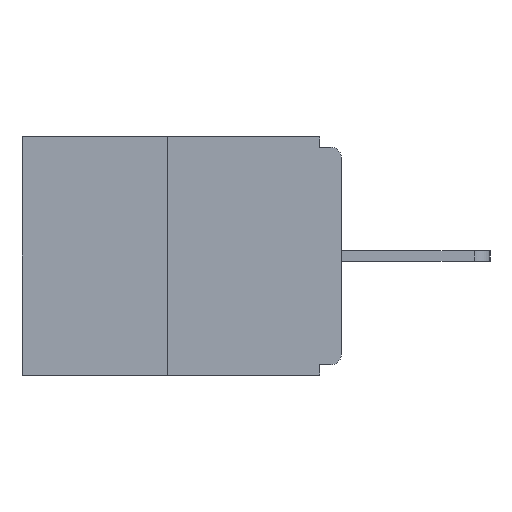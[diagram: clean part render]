
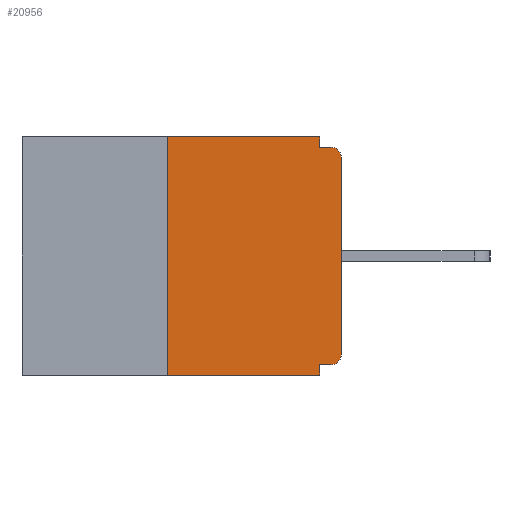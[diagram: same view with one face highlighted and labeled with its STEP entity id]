
A CAD part, left-side view. The second image highlights one B-rep face of the part: STEP entity #20956.
In plain terms, the highlighted planar face has unit normal (-1, 0, 0).
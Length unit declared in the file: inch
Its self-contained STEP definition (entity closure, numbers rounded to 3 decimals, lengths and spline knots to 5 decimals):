
#208 = PLANE ( 'NONE',  #18270 ) ;
#261 = ORIENTED_EDGE ( 'NONE', *, *, #8516, .T. ) ;
#302 = DIRECTION ( 'NONE',  ( 0., 0., -1. ) ) ;
#367 = VERTEX_POINT ( 'NONE', #8144 ) ;
#440 = DIRECTION ( 'NONE',  ( -1., 0., 0. ) ) ;
#805 = ORIENTED_EDGE ( 'NONE', *, *, #15250, .F. ) ;
#1220 = VECTOR ( 'NONE', #7084, 39.37008 ) ;
#1241 = EDGE_CURVE ( 'NONE', #21576, #4973, #9445, .T. ) ;
#1462 = CARTESIAN_POINT ( 'NONE',  ( 0., 0., -0.328 ) ) ;
#1525 = VECTOR ( 'NONE', #11750, 39.37008 ) ;
#1815 = CARTESIAN_POINT ( 'NONE',  ( 0., 0.46, -0.343 ) ) ;
#1885 = LINE ( 'NONE', #5015, #1220 ) ;
#2159 = VERTEX_POINT ( 'NONE', #21893 ) ;
#2286 = CARTESIAN_POINT ( 'NONE',  ( 0., 0., -0.313 ) ) ;
#2375 = CIRCLE ( 'NONE', #11720, 0.015 ) ;
#2569 = DIRECTION ( 'NONE',  ( 0., -1., 0. ) ) ;
#2678 = DIRECTION ( 'NONE',  ( -1., 0., 0. ) ) ;
#2682 = CARTESIAN_POINT ( 'NONE',  ( 0., 0.015, -0.03 ) ) ;
#3035 = DIRECTION ( 'NONE',  ( 0., 0., -1. ) ) ;
#3646 = VERTEX_POINT ( 'NONE', #17902 ) ;
#3675 = VERTEX_POINT ( 'NONE', #14904 ) ;
#3865 = EDGE_CURVE ( 'NONE', #11696, #3646, #16246, .T. ) ;
#4029 = EDGE_CURVE ( 'NONE', #2159, #4973, #11850, .T. ) ;
#4383 = EDGE_CURVE ( 'NONE', #3646, #3675, #14090, .T. ) ;
#4403 = DIRECTION ( 'NONE',  ( 0., 0., 1. ) ) ;
#4973 = VERTEX_POINT ( 'NONE', #11235 ) ;
#5015 = CARTESIAN_POINT ( 'NONE',  ( 0., 0.46, 0. ) ) ;
#5054 = CARTESIAN_POINT ( 'NONE',  ( 0., 0., 0. ) ) ;
#5419 = EDGE_CURVE ( 'NONE', #2159, #21942, #5469, .T. ) ;
#5469 = LINE ( 'NONE', #5859, #17418 ) ;
#5816 = FACE_OUTER_BOUND ( 'NONE', #8171, .T. ) ;
#5859 = CARTESIAN_POINT ( 'NONE',  ( 0., 0.25, 0. ) ) ;
#5953 = DIRECTION ( 'NONE',  ( 0., 0., 1. ) ) ;
#6061 = CARTESIAN_POINT ( 'NONE',  ( 0., 0.25, 0. ) ) ;
#6638 = ORIENTED_EDGE ( 'NONE', *, *, #5419, .F. ) ;
#7041 = CARTESIAN_POINT ( 'NONE',  ( 0., 0.015, -0.328 ) ) ;
#7084 = DIRECTION ( 'NONE',  ( 0., -1., 0. ) ) ;
#8128 = DIRECTION ( 'NONE',  ( 0., -1., 0. ) ) ;
#8144 = CARTESIAN_POINT ( 'NONE',  ( 0., 0.031, 0. ) ) ;
#8171 = EDGE_LOOP ( 'NONE', ( #13307, #6638, #11545, #25589, #24665, #261, #10083, #9889, #805, #13201 ) ) ;
#8516 = EDGE_CURVE ( 'NONE', #13778, #11696, #2375, .T. ) ;
#8519 = CARTESIAN_POINT ( 'NONE',  ( 0., 0.46, 0. ) ) ;
#8806 = VERTEX_POINT ( 'NONE', #19523 ) ;
#9445 = LINE ( 'NONE', #21220, #18177 ) ;
#9889 = ORIENTED_EDGE ( 'NONE', *, *, #4383, .T. ) ;
#10083 = ORIENTED_EDGE ( 'NONE', *, *, #3865, .T. ) ;
#11235 = CARTESIAN_POINT ( 'NONE',  ( 0., 0.031, -0.343 ) ) ;
#11545 = ORIENTED_EDGE ( 'NONE', *, *, #4029, .T. ) ;
#11673 = CARTESIAN_POINT ( 'NONE',  ( 0., 0.031, 0. ) ) ;
#11696 = VERTEX_POINT ( 'NONE', #2286 ) ;
#11720 = AXIS2_PLACEMENT_3D ( 'NONE', #12731, #440, #14732 ) ;
#11750 = DIRECTION ( 'NONE',  ( 0., 1., 0. ) ) ;
#11850 = LINE ( 'NONE', #1815, #21709 ) ;
#12601 = DIRECTION ( 'NONE',  ( 1., 0., 0. ) ) ;
#12731 = CARTESIAN_POINT ( 'NONE',  ( 0., 0.015, -0.313 ) ) ;
#12758 = CARTESIAN_POINT ( 'NONE',  ( 0., 0., -0.015 ) ) ;
#12910 = CARTESIAN_POINT ( 'NONE',  ( 0., 0.031, -0.328 ) ) ;
#13201 = ORIENTED_EDGE ( 'NONE', *, *, #23202, .F. ) ;
#13307 = ORIENTED_EDGE ( 'NONE', *, *, #22850, .F. ) ;
#13778 = VERTEX_POINT ( 'NONE', #7041 ) ;
#13983 = VECTOR ( 'NONE', #23412, 39.37008 ) ;
#14090 = CIRCLE ( 'NONE', #19981, 0.015 ) ;
#14732 = DIRECTION ( 'NONE',  ( 0., 0., -1. ) ) ;
#14904 = CARTESIAN_POINT ( 'NONE',  ( 0., 0.015, -0.015 ) ) ;
#15250 = EDGE_CURVE ( 'NONE', #8806, #3675, #18335, .T. ) ;
#16246 = LINE ( 'NONE', #5054, #20234 ) ;
#17418 = VECTOR ( 'NONE', #5953, 39.37008 ) ;
#17706 = VECTOR ( 'NONE', #2569, 39.37008 ) ;
#17902 = CARTESIAN_POINT ( 'NONE',  ( 0., 0., -0.03 ) ) ;
#18177 = VECTOR ( 'NONE', #20975, 39.37008 ) ;
#18270 = AXIS2_PLACEMENT_3D ( 'NONE', #8519, #12601, #302 ) ;
#18307 = LINE ( 'NONE', #1462, #1525 ) ;
#18335 = LINE ( 'NONE', #12758, #17706 ) ;
#19523 = CARTESIAN_POINT ( 'NONE',  ( 0., 0.031, -0.015 ) ) ;
#19981 = AXIS2_PLACEMENT_3D ( 'NONE', #2682, #2678, #3035 ) ;
#20234 = VECTOR ( 'NONE', #4403, 39.37008 ) ;
#20956 = ADVANCED_FACE ( 'NONE', ( #5816 ), #208, .F. ) ;
#20975 = DIRECTION ( 'NONE',  ( 0., 0., -1. ) ) ;
#21220 = CARTESIAN_POINT ( 'NONE',  ( 0., 0.031, -0.343 ) ) ;
#21576 = VERTEX_POINT ( 'NONE', #12910 ) ;
#21709 = VECTOR ( 'NONE', #8128, 39.37008 ) ;
#21893 = CARTESIAN_POINT ( 'NONE',  ( 0., 0.25, -0.343 ) ) ;
#21942 = VERTEX_POINT ( 'NONE', #6061 ) ;
#22850 = EDGE_CURVE ( 'NONE', #21942, #367, #1885, .T. ) ;
#23044 = EDGE_CURVE ( 'NONE', #13778, #21576, #18307, .T. ) ;
#23202 = EDGE_CURVE ( 'NONE', #367, #8806, #23730, .T. ) ;
#23412 = DIRECTION ( 'NONE',  ( 0., 0., -1. ) ) ;
#23730 = LINE ( 'NONE', #11673, #13983 ) ;
#24665 = ORIENTED_EDGE ( 'NONE', *, *, #23044, .F. ) ;
#25589 = ORIENTED_EDGE ( 'NONE', *, *, #1241, .F. ) ;
